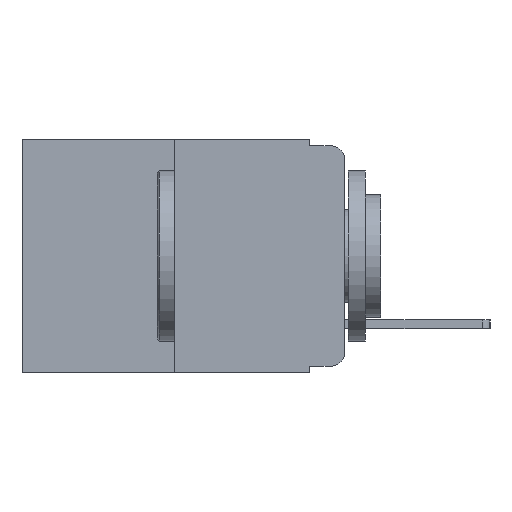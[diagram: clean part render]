
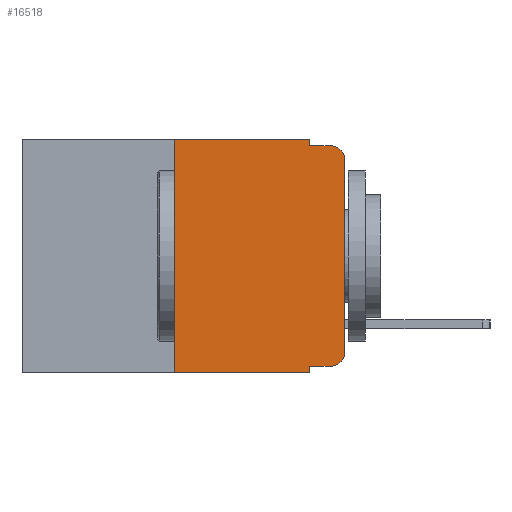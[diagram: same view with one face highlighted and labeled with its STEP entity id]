
A CAD part, left-side view. The second image highlights one B-rep face of the part: STEP entity #16518.
In plain terms, the highlighted planar face has unit normal (-1, 0, 0).
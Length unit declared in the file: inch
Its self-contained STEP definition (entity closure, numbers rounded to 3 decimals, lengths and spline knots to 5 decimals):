
#28 = VECTOR ( 'NONE', #1706, 39.37008 ) ;
#82 = DIRECTION ( 'NONE',  ( 0., 0., -1. ) ) ;
#110 = CARTESIAN_POINT ( 'NONE',  ( 0., 0.051, -0.01 ) ) ;
#627 = DIRECTION ( 'NONE',  ( -1., 0., 0. ) ) ;
#921 = EDGE_CURVE ( 'NONE', #15742, #10749, #11390, .T. ) ;
#935 = CARTESIAN_POINT ( 'NONE',  ( 0., 0.051, -0.333 ) ) ;
#1277 = EDGE_CURVE ( 'NONE', #15742, #15483, #14024, .T. ) ;
#1706 = DIRECTION ( 'NONE',  ( 0., 0., 1. ) ) ;
#1984 = EDGE_CURVE ( 'NONE', #15483, #12028, #12903, .T. ) ;
#2089 = EDGE_LOOP ( 'NONE', ( #12892, #2287, #18335, #7981, #11789, #5017, #17257, #6841, #10674, #7766 ) ) ;
#2287 = ORIENTED_EDGE ( 'NONE', *, *, #13101, .T. ) ;
#2329 = DIRECTION ( 'NONE',  ( -1., 0., 0. ) ) ;
#2609 = DIRECTION ( 'NONE',  ( 0., 0., -1. ) ) ;
#2659 = VECTOR ( 'NONE', #17219, 39.37008 ) ;
#3078 = AXIS2_PLACEMENT_3D ( 'NONE', #16841, #11261, #2609 ) ;
#3194 = VECTOR ( 'NONE', #9742, 39.37008 ) ;
#3548 = VECTOR ( 'NONE', #3927, 39.37008 ) ;
#3701 = VECTOR ( 'NONE', #8078, 39.37008 ) ;
#3853 = LINE ( 'NONE', #15974, #28 ) ;
#3927 = DIRECTION ( 'NONE',  ( 0., 0., 1. ) ) ;
#4223 = CARTESIAN_POINT ( 'NONE',  ( 0., 0.051, -0.333 ) ) ;
#4776 = VERTEX_POINT ( 'NONE', #6558 ) ;
#5017 = ORIENTED_EDGE ( 'NONE', *, *, #10736, .F. ) ;
#5348 = DIRECTION ( 'NONE',  ( 0., -1., 0. ) ) ;
#5433 = CARTESIAN_POINT ( 'NONE',  ( 0., 0.25, -0.343 ) ) ;
#5452 = PLANE ( 'NONE',  #3078 ) ;
#5617 = VECTOR ( 'NONE', #5348, 39.37008 ) ;
#5980 = DIRECTION ( 'NONE',  ( 0., -1., 0. ) ) ;
#6558 = CARTESIAN_POINT ( 'NONE',  ( 0., 0., -0.03 ) ) ;
#6841 = ORIENTED_EDGE ( 'NONE', *, *, #921, .F. ) ;
#6948 = CARTESIAN_POINT ( 'NONE',  ( 0., 0.02, -0.01 ) ) ;
#7766 = ORIENTED_EDGE ( 'NONE', *, *, #1984, .T. ) ;
#7916 = CARTESIAN_POINT ( 'NONE',  ( 0., 0.051, 0. ) ) ;
#7981 = ORIENTED_EDGE ( 'NONE', *, *, #10631, .F. ) ;
#8078 = DIRECTION ( 'NONE',  ( 0., 0., -1. ) ) ;
#8962 = CARTESIAN_POINT ( 'NONE',  ( 0., 0.25, 0. ) ) ;
#9282 = CARTESIAN_POINT ( 'NONE',  ( 0., 0.02, -0.313 ) ) ;
#9365 = VECTOR ( 'NONE', #5980, 39.37008 ) ;
#9380 = VERTEX_POINT ( 'NONE', #6948 ) ;
#9471 = LINE ( 'NONE', #13935, #5617 ) ;
#9742 = DIRECTION ( 'NONE',  ( 0., -1., 0. ) ) ;
#9801 = CARTESIAN_POINT ( 'NONE',  ( 0., 0.473, 0. ) ) ;
#9937 = CIRCLE ( 'NONE', #10032, 0.02 ) ;
#10032 = AXIS2_PLACEMENT_3D ( 'NONE', #10993, #2329, #12416 ) ;
#10295 = CARTESIAN_POINT ( 'NONE',  ( 0., 0.051, -0.01 ) ) ;
#10420 = LINE ( 'NONE', #9801, #3194 ) ;
#10631 = EDGE_CURVE ( 'NONE', #13297, #18147, #16588, .T. ) ;
#10674 = ORIENTED_EDGE ( 'NONE', *, *, #1277, .T. ) ;
#10715 = DIRECTION ( 'NONE',  ( 0., 0., -1. ) ) ;
#10736 = EDGE_CURVE ( 'NONE', #15273, #16972, #3853, .T. ) ;
#10749 = VERTEX_POINT ( 'NONE', #11807 ) ;
#10993 = CARTESIAN_POINT ( 'NONE',  ( 0., 0.02, -0.03 ) ) ;
#11261 = DIRECTION ( 'NONE',  ( 1., 0., 0. ) ) ;
#11390 = LINE ( 'NONE', #7916, #3701 ) ;
#11564 = CARTESIAN_POINT ( 'NONE',  ( 0., 0.051, 0. ) ) ;
#11789 = ORIENTED_EDGE ( 'NONE', *, *, #12662, .F. ) ;
#11807 = CARTESIAN_POINT ( 'NONE',  ( 0., 0.051, -0.343 ) ) ;
#11952 = EDGE_CURVE ( 'NONE', #15273, #10749, #9471, .T. ) ;
#12028 = VERTEX_POINT ( 'NONE', #14051 ) ;
#12416 = DIRECTION ( 'NONE',  ( 0., 0., -1. ) ) ;
#12561 = CARTESIAN_POINT ( 'NONE',  ( 0., 0., 0. ) ) ;
#12662 = EDGE_CURVE ( 'NONE', #16972, #13297, #10420, .T. ) ;
#12870 = VECTOR ( 'NONE', #82, 39.37008 ) ;
#12892 = ORIENTED_EDGE ( 'NONE', *, *, #14708, .T. ) ;
#12903 = CIRCLE ( 'NONE', #18194, 0.02 ) ;
#13101 = EDGE_CURVE ( 'NONE', #4776, #9380, #9937, .T. ) ;
#13170 = CARTESIAN_POINT ( 'NONE',  ( 0., 0.02, -0.333 ) ) ;
#13297 = VERTEX_POINT ( 'NONE', #18445 ) ;
#13935 = CARTESIAN_POINT ( 'NONE',  ( 0., 0.473, -0.343 ) ) ;
#14024 = LINE ( 'NONE', #4223, #9365 ) ;
#14051 = CARTESIAN_POINT ( 'NONE',  ( 0., 0., -0.313 ) ) ;
#14315 = EDGE_CURVE ( 'NONE', #18147, #9380, #18240, .T. ) ;
#14539 = LINE ( 'NONE', #12561, #3548 ) ;
#14708 = EDGE_CURVE ( 'NONE', #12028, #4776, #14539, .T. ) ;
#15273 = VERTEX_POINT ( 'NONE', #5433 ) ;
#15483 = VERTEX_POINT ( 'NONE', #13170 ) ;
#15742 = VERTEX_POINT ( 'NONE', #935 ) ;
#15974 = CARTESIAN_POINT ( 'NONE',  ( 0., 0.25, 0. ) ) ;
#16518 = ADVANCED_FACE ( 'NONE', ( #16672 ), #5452, .F. ) ;
#16588 = LINE ( 'NONE', #11564, #12870 ) ;
#16672 = FACE_OUTER_BOUND ( 'NONE', #2089, .T. ) ;
#16841 = CARTESIAN_POINT ( 'NONE',  ( 0., 0.473, 0. ) ) ;
#16972 = VERTEX_POINT ( 'NONE', #8962 ) ;
#17219 = DIRECTION ( 'NONE',  ( 0., -1., 0. ) ) ;
#17257 = ORIENTED_EDGE ( 'NONE', *, *, #11952, .T. ) ;
#18147 = VERTEX_POINT ( 'NONE', #10295 ) ;
#18194 = AXIS2_PLACEMENT_3D ( 'NONE', #9282, #627, #10715 ) ;
#18240 = LINE ( 'NONE', #110, #2659 ) ;
#18335 = ORIENTED_EDGE ( 'NONE', *, *, #14315, .F. ) ;
#18445 = CARTESIAN_POINT ( 'NONE',  ( 0., 0.051, 0. ) ) ;
